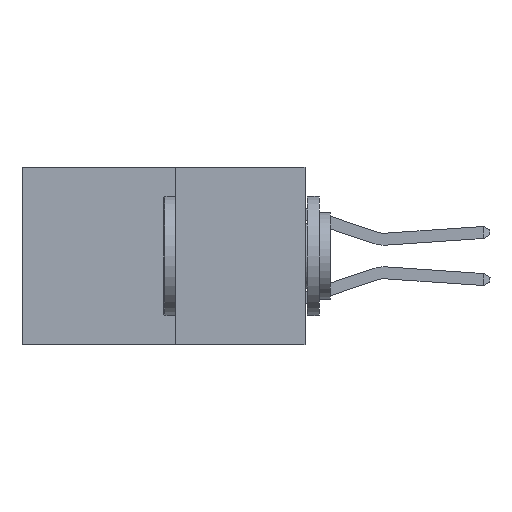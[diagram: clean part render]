
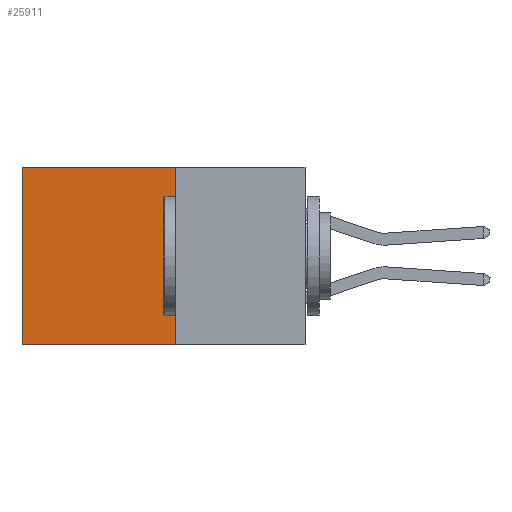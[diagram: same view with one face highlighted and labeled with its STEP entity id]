
A CAD part, left-side view. The second image highlights one B-rep face of the part: STEP entity #25911.
In plain terms, the highlighted planar face has unit normal (-1, 0, 0).
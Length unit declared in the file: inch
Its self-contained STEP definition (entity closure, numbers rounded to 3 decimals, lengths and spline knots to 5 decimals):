
#1703 = CARTESIAN_POINT ( 'NONE',  ( 0.277, 0.27, 0. ) ) ;
#2617 = EDGE_LOOP ( 'NONE', ( #28567, #10604, #3575, #4577 ) ) ;
#3292 = DIRECTION ( 'NONE',  ( 0., 1., 0. ) ) ;
#3575 = ORIENTED_EDGE ( 'NONE', *, *, #15559, .F. ) ;
#4577 = ORIENTED_EDGE ( 'NONE', *, *, #27546, .T. ) ;
#5965 = CARTESIAN_POINT ( 'NONE',  ( 0.277, 0.27, -0.37 ) ) ;
#7185 = CARTESIAN_POINT ( 'NONE',  ( 0.277, 0.27, -0.37 ) ) ;
#7762 = CARTESIAN_POINT ( 'NONE',  ( 0.277, 0.59, -0.37 ) ) ;
#8096 = VECTOR ( 'NONE', #20762, 39.37008 ) ;
#8445 = CARTESIAN_POINT ( 'NONE',  ( 0.277, 0.27, 0. ) ) ;
#8944 = AXIS2_PLACEMENT_3D ( 'NONE', #25896, #33771, #18148 ) ;
#9868 = VERTEX_POINT ( 'NONE', #1703 ) ;
#9889 = FACE_OUTER_BOUND ( 'NONE', #2617, .T. ) ;
#10604 = ORIENTED_EDGE ( 'NONE', *, *, #13313, .F. ) ;
#10687 = LINE ( 'NONE', #16602, #30769 ) ;
#10926 = VERTEX_POINT ( 'NONE', #5965 ) ;
#13313 = EDGE_CURVE ( 'NONE', #10926, #21227, #10687, .T. ) ;
#15057 = LINE ( 'NONE', #7762, #8096 ) ;
#15559 = EDGE_CURVE ( 'NONE', #9868, #10926, #18794, .T. ) ;
#16602 = CARTESIAN_POINT ( 'NONE',  ( 0.277, 0.27, -0.37 ) ) ;
#18148 = DIRECTION ( 'NONE',  ( 0., 0., -1. ) ) ;
#18794 = LINE ( 'NONE', #7185, #27496 ) ;
#20762 = DIRECTION ( 'NONE',  ( 0., 0., -1. ) ) ;
#21227 = VERTEX_POINT ( 'NONE', #30295 ) ;
#22054 = VECTOR ( 'NONE', #3292, 39.37008 ) ;
#25896 = CARTESIAN_POINT ( 'NONE',  ( 0.277, 0.27, -0.37 ) ) ;
#25911 = ADVANCED_FACE ( 'NONE', ( #9889 ), #31206, .F. ) ;
#27087 = DIRECTION ( 'NONE',  ( 0., 1., 0. ) ) ;
#27214 = VERTEX_POINT ( 'NONE', #30788 ) ;
#27496 = VECTOR ( 'NONE', #28131, 39.37008 ) ;
#27546 = EDGE_CURVE ( 'NONE', #9868, #27214, #29897, .T. ) ;
#28131 = DIRECTION ( 'NONE',  ( 0., 0., -1. ) ) ;
#28567 = ORIENTED_EDGE ( 'NONE', *, *, #30933, .T. ) ;
#29897 = LINE ( 'NONE', #8445, #22054 ) ;
#30295 = CARTESIAN_POINT ( 'NONE',  ( 0.277, 0.59, -0.37 ) ) ;
#30769 = VECTOR ( 'NONE', #27087, 39.37008 ) ;
#30788 = CARTESIAN_POINT ( 'NONE',  ( 0.277, 0.59, 0. ) ) ;
#30933 = EDGE_CURVE ( 'NONE', #27214, #21227, #15057, .T. ) ;
#31206 = PLANE ( 'NONE',  #8944 ) ;
#33771 = DIRECTION ( 'NONE',  ( 1., 0., 0. ) ) ;
